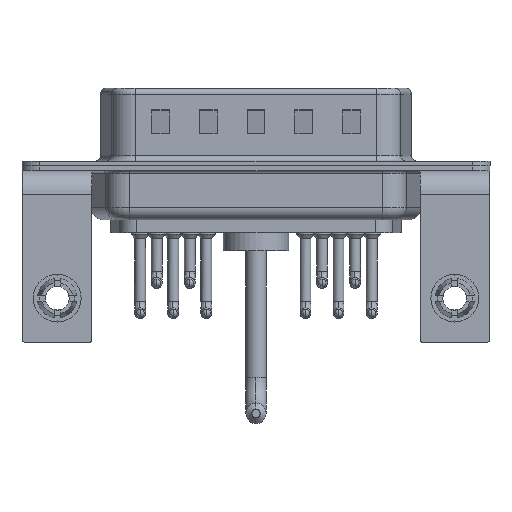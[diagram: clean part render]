
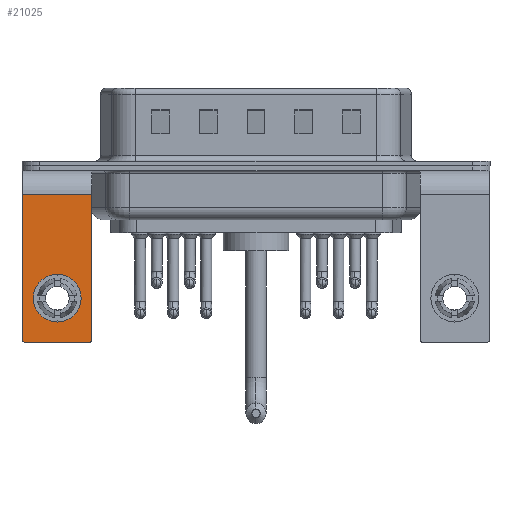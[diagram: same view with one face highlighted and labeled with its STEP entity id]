
A CAD part, front view. The second image highlights one B-rep face of the part: STEP entity #21025.
In plain terms, the highlighted planar face has unit normal (0, -1, 0).
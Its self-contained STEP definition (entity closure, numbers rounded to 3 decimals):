
#5 = DIRECTION ( 'NONE',  ( 0., 1., 0. ) ) ;
#690 = AXIS2_PLACEMENT_3D ( 'NONE', #10111, #4733, #21757 ) ;
#697 = ORIENTED_EDGE ( 'NONE', *, *, #13394, .T. ) ;
#729 = CARTESIAN_POINT ( 'NONE',  ( -2.9, -6.25, -2.4 ) ) ;
#730 = VECTOR ( 'NONE', #18504, 1000. ) ;
#934 = DIRECTION ( 'NONE',  ( 0., 1., 0. ) ) ;
#1089 = CARTESIAN_POINT ( 'NONE',  ( 2.9, -6.25, -2.4 ) ) ;
#1144 = CIRCLE ( 'NONE', #18752, 2. ) ;
#1897 = CIRCLE ( 'NONE', #690, 0.25 ) ;
#2051 = AXIS2_PLACEMENT_3D ( 'NONE', #1089, #14365, #16750 ) ;
#2972 = EDGE_LOOP ( 'NONE', ( #697, #22708, #6897, #17522, #19574, #9892 ) ) ;
#3120 = CARTESIAN_POINT ( 'NONE',  ( 2.9, -6.25, -2.4 ) ) ;
#3266 = EDGE_CURVE ( 'NONE', #22240, #9937, #1897, .T. ) ;
#3303 = VERTEX_POINT ( 'NONE', #729 ) ;
#3447 = DIRECTION ( 'NONE',  ( 0., -1., 0. ) ) ;
#3684 = DIRECTION ( 'NONE',  ( 0., 0., 1. ) ) ;
#3701 = AXIS2_PLACEMENT_3D ( 'NONE', #22089, #934, #23847 ) ;
#4029 = CARTESIAN_POINT ( 'NONE',  ( 2.9, -6.25, -14.8 ) ) ;
#4695 = CARTESIAN_POINT ( 'NONE',  ( 2.9, -6.25, -14.55 ) ) ;
#4733 = DIRECTION ( 'NONE',  ( 0., -1., 0. ) ) ;
#5361 = VERTEX_POINT ( 'NONE', #14984 ) ;
#6100 = CARTESIAN_POINT ( 'NONE',  ( -2.9, -6.25, -14.55 ) ) ;
#6897 = ORIENTED_EDGE ( 'NONE', *, *, #13176, .F. ) ;
#6938 = VECTOR ( 'NONE', #16262, 1000. ) ;
#7545 = DIRECTION ( 'NONE',  ( 0., 0., 1. ) ) ;
#8020 = CARTESIAN_POINT ( 'NONE',  ( -2.9, -6.25, -2.4 ) ) ;
#8148 = VERTEX_POINT ( 'NONE', #6100 ) ;
#8159 = VERTEX_POINT ( 'NONE', #10347 ) ;
#8378 = VERTEX_POINT ( 'NONE', #18490 ) ;
#8736 = LINE ( 'NONE', #3120, #6938 ) ;
#9106 = FACE_BOUND ( 'NONE', #20104, .T. ) ;
#9665 = ORIENTED_EDGE ( 'NONE', *, *, #16845, .T. ) ;
#9892 = ORIENTED_EDGE ( 'NONE', *, *, #22294, .T. ) ;
#9937 = VERTEX_POINT ( 'NONE', #4695 ) ;
#10033 = EDGE_CURVE ( 'NONE', #24384, #8159, #10869, .T. ) ;
#10111 = CARTESIAN_POINT ( 'NONE',  ( 2.65, -6.25, -14.55 ) ) ;
#10347 = CARTESIAN_POINT ( 'NONE',  ( 0., -6.25, -9.07 ) ) ;
#10509 = AXIS2_PLACEMENT_3D ( 'NONE', #14961, #3447, #3684 ) ;
#10730 = CARTESIAN_POINT ( 'NONE',  ( 2.9, -6.25, -2.4 ) ) ;
#10843 = FACE_OUTER_BOUND ( 'NONE', #2972, .T. ) ;
#10869 = CIRCLE ( 'NONE', #3701, 2. ) ;
#12282 = LINE ( 'NONE', #8020, #16230 ) ;
#13176 = EDGE_CURVE ( 'NONE', #22240, #8378, #14945, .T. ) ;
#13394 = EDGE_CURVE ( 'NONE', #3303, #8148, #12282, .T. ) ;
#13949 = EDGE_CURVE ( 'NONE', #5361, #9937, #8736, .T. ) ;
#14365 = DIRECTION ( 'NONE',  ( 0., 1., 0. ) ) ;
#14765 = CARTESIAN_POINT ( 'NONE',  ( 2.65, -6.25, -14.8 ) ) ;
#14945 = LINE ( 'NONE', #4029, #23816 ) ;
#14961 = CARTESIAN_POINT ( 'NONE',  ( -2.65, -6.25, -14.55 ) ) ;
#14984 = CARTESIAN_POINT ( 'NONE',  ( 2.9, -6.25, -2.4 ) ) ;
#15907 = DIRECTION ( 'NONE',  ( 0., 0., -1. ) ) ;
#16230 = VECTOR ( 'NONE', #15907, 1000. ) ;
#16262 = DIRECTION ( 'NONE',  ( 0., 0., -1. ) ) ;
#16277 = ORIENTED_EDGE ( 'NONE', *, *, #10033, .T. ) ;
#16492 = PLANE ( 'NONE',  #2051 ) ;
#16750 = DIRECTION ( 'NONE',  ( 0., 0., 1. ) ) ;
#16845 = EDGE_CURVE ( 'NONE', #8159, #24384, #1144, .T. ) ;
#17522 = ORIENTED_EDGE ( 'NONE', *, *, #3266, .T. ) ;
#17696 = CARTESIAN_POINT ( 'NONE',  ( 0., -6.25, -13.07 ) ) ;
#18490 = CARTESIAN_POINT ( 'NONE',  ( -2.65, -6.25, -14.8 ) ) ;
#18504 = DIRECTION ( 'NONE',  ( -1., 0., 0. ) ) ;
#18752 = AXIS2_PLACEMENT_3D ( 'NONE', #24441, #5, #7545 ) ;
#19574 = ORIENTED_EDGE ( 'NONE', *, *, #13949, .F. ) ;
#20052 = CIRCLE ( 'NONE', #10509, 0.25 ) ;
#20104 = EDGE_LOOP ( 'NONE', ( #16277, #9665 ) ) ;
#21025 = ADVANCED_FACE ( 'NONE', ( #9106, #10843 ), #16492, .F. ) ;
#21757 = DIRECTION ( 'NONE',  ( 0., 0., 1. ) ) ;
#22089 = CARTESIAN_POINT ( 'NONE',  ( 0., -6.25, -11.07 ) ) ;
#22240 = VERTEX_POINT ( 'NONE', #14765 ) ;
#22264 = LINE ( 'NONE', #10730, #730 ) ;
#22294 = EDGE_CURVE ( 'NONE', #5361, #3303, #22264, .T. ) ;
#22708 = ORIENTED_EDGE ( 'NONE', *, *, #24672, .T. ) ;
#23816 = VECTOR ( 'NONE', #24700, 1000. ) ;
#23847 = DIRECTION ( 'NONE',  ( 0., 0., 1. ) ) ;
#24384 = VERTEX_POINT ( 'NONE', #17696 ) ;
#24441 = CARTESIAN_POINT ( 'NONE',  ( 0., -6.25, -11.07 ) ) ;
#24672 = EDGE_CURVE ( 'NONE', #8148, #8378, #20052, .T. ) ;
#24700 = DIRECTION ( 'NONE',  ( -1., 0., 0. ) ) ;
